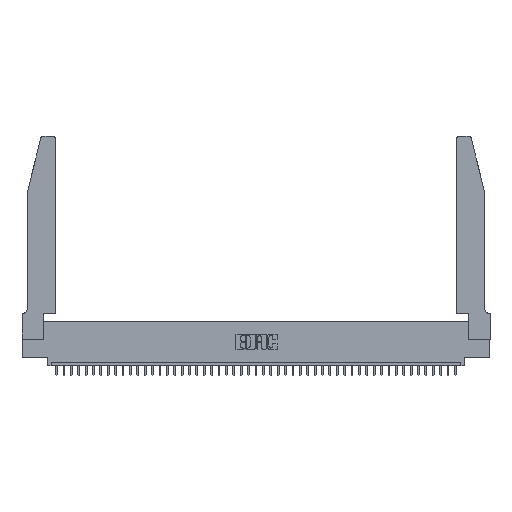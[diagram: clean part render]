
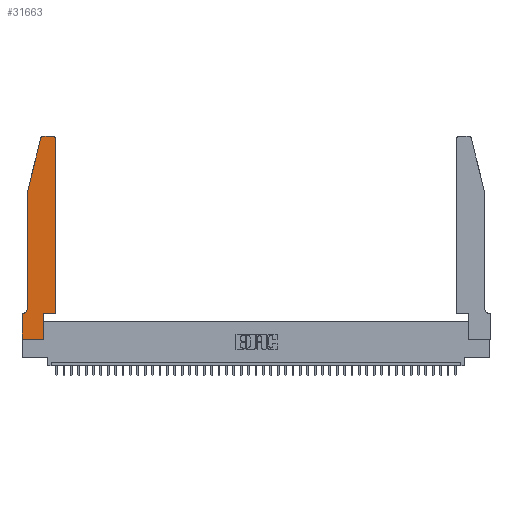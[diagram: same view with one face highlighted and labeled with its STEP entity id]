
A CAD part, top view. The second image highlights one B-rep face of the part: STEP entity #31663.
In plain terms, the highlighted planar face has unit normal (0, 0, 1).
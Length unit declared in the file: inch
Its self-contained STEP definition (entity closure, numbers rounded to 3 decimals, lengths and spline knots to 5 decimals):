
#467 = LINE ( 'NONE', #30379, #32256 ) ;
#498 = EDGE_CURVE ( 'NONE', #43970, #18253, #39390, .T. ) ;
#1003 = FACE_OUTER_BOUND ( 'NONE', #10533, .T. ) ;
#1211 = CIRCLE ( 'NONE', #13735, 0.07 ) ;
#1346 = DIRECTION ( 'NONE',  ( 1., 0., 0. ) ) ;
#2030 = DIRECTION ( 'NONE',  ( 0., 0., -1. ) ) ;
#2126 = EDGE_CURVE ( 'NONE', #4082, #16941, #1211, .T. ) ;
#2591 = CARTESIAN_POINT ( 'NONE',  ( 0.0055, 0.35, 0.37 ) ) ;
#3167 = EDGE_CURVE ( 'NONE', #43345, #43970, #38235, .T. ) ;
#3253 = CARTESIAN_POINT ( 'NONE',  ( 0.2605, 2.75, 0.37 ) ) ;
#3808 = ORIENTED_EDGE ( 'NONE', *, *, #30053, .T. ) ;
#3854 = VECTOR ( 'NONE', #9571, 39.37008 ) ;
#4082 = VERTEX_POINT ( 'NONE', #9560 ) ;
#4664 = DIRECTION ( 'NONE',  ( 0., 1., 0. ) ) ;
#5843 = CARTESIAN_POINT ( 'NONE',  ( 0., 0.35, 0.37 ) ) ;
#6270 = CARTESIAN_POINT ( 'NONE',  ( 0., 0., 0.37 ) ) ;
#9437 = DIRECTION ( 'NONE',  ( 1., 0., 0. ) ) ;
#9560 = CARTESIAN_POINT ( 'NONE',  ( 0.0755, 0.42, 0.37 ) ) ;
#9571 = DIRECTION ( 'NONE',  ( 1., 0., 0. ) ) ;
#10533 = EDGE_LOOP ( 'NONE', ( #23022, #24899, #38651, #12901, #29548, #28961, #37456, #3808, #36586, #33849, #40538, #20449 ) ) ;
#12121 = DIRECTION ( 'NONE',  ( -1., 0., 0. ) ) ;
#12220 = EDGE_CURVE ( 'NONE', #16941, #22167, #467, .T. ) ;
#12901 = ORIENTED_EDGE ( 'NONE', *, *, #14897, .T. ) ;
#13027 = PLANE ( 'NONE',  #43743 ) ;
#13198 = DIRECTION ( 'NONE',  ( 1., 0., 0. ) ) ;
#13690 = CARTESIAN_POINT ( 'NONE',  ( 0.25487, 2.72718, 0.37 ) ) ;
#13735 = AXIS2_PLACEMENT_3D ( 'NONE', #22420, #2030, #12121 ) ;
#13819 = CARTESIAN_POINT ( 'NONE',  ( 0.2865, 0., 0.37 ) ) ;
#14368 = CARTESIAN_POINT ( 'NONE',  ( 0., 0., 0.37 ) ) ;
#14806 = CIRCLE ( 'NONE', #32439, 0.03 ) ;
#14897 = EDGE_CURVE ( 'NONE', #21212, #4082, #32716, .T. ) ;
#15145 = LINE ( 'NONE', #40235, #21542 ) ;
#15285 = CARTESIAN_POINT ( 'NONE',  ( 0., 0., 0.37 ) ) ;
#15328 = CARTESIAN_POINT ( 'NONE',  ( 0.4505, 0.35, 0.37 ) ) ;
#16217 = LINE ( 'NONE', #35385, #42052 ) ;
#16904 = VERTEX_POINT ( 'NONE', #15285 ) ;
#16941 = VERTEX_POINT ( 'NONE', #2591 ) ;
#18173 = LINE ( 'NONE', #21728, #39775 ) ;
#18253 = VERTEX_POINT ( 'NONE', #13690 ) ;
#19038 = LINE ( 'NONE', #20580, #34201 ) ;
#19192 = EDGE_CURVE ( 'NONE', #38780, #36599, #15145, .T. ) ;
#20449 = ORIENTED_EDGE ( 'NONE', *, *, #27461, .T. ) ;
#20580 = CARTESIAN_POINT ( 'NONE',  ( 0.4505, 0.35, 0.37 ) ) ;
#21212 = VERTEX_POINT ( 'NONE', #39791 ) ;
#21542 = VECTOR ( 'NONE', #24767, 39.37008 ) ;
#21728 = CARTESIAN_POINT ( 'NONE',  ( 0.4505, 0.35, 0.37 ) ) ;
#21789 = DIRECTION ( 'NONE',  ( -0.239, -0.971, 0. ) ) ;
#21903 = DIRECTION ( 'NONE',  ( 0., 0., 1. ) ) ;
#22167 = VERTEX_POINT ( 'NONE', #43435 ) ;
#22420 = CARTESIAN_POINT ( 'NONE',  ( 0.0055, 0.42, 0.37 ) ) ;
#22748 = LINE ( 'NONE', #14368, #40016 ) ;
#23022 = ORIENTED_EDGE ( 'NONE', *, *, #3167, .T. ) ;
#23061 = EDGE_CURVE ( 'NONE', #18253, #21212, #16217, .T. ) ;
#23567 = VECTOR ( 'NONE', #38788, 39.37008 ) ;
#24750 = VECTOR ( 'NONE', #27511, 39.37008 ) ;
#24767 = DIRECTION ( 'NONE',  ( 0., 1., 0. ) ) ;
#24899 = ORIENTED_EDGE ( 'NONE', *, *, #498, .T. ) ;
#25700 = CARTESIAN_POINT ( 'NONE',  ( 0.284, 2.72, 0.37 ) ) ;
#26692 = DIRECTION ( 'NONE',  ( 0., 0., 1. ) ) ;
#27052 = DIRECTION ( 'NONE',  ( 1., 0., 0. ) ) ;
#27073 = VERTEX_POINT ( 'NONE', #38041 ) ;
#27461 = EDGE_CURVE ( 'NONE', #27073, #43345, #14806, .T. ) ;
#27511 = DIRECTION ( 'NONE',  ( -1., 0., 0. ) ) ;
#28961 = ORIENTED_EDGE ( 'NONE', *, *, #12220, .T. ) ;
#29004 = CARTESIAN_POINT ( 'NONE',  ( 0.0755, 2., 0.37 ) ) ;
#29036 = VERTEX_POINT ( 'NONE', #15328 ) ;
#29548 = ORIENTED_EDGE ( 'NONE', *, *, #2126, .T. ) ;
#30053 = EDGE_CURVE ( 'NONE', #16904, #38780, #31781, .T. ) ;
#30379 = CARTESIAN_POINT ( 'NONE',  ( 0.0755, 0.35, 0.37 ) ) ;
#31663 = ADVANCED_FACE ( 'NONE', ( #1003 ), #13027, .T. ) ;
#31781 = LINE ( 'NONE', #6270, #3854 ) ;
#32256 = VECTOR ( 'NONE', #33854, 39.37008 ) ;
#32439 = AXIS2_PLACEMENT_3D ( 'NONE', #36181, #26692, #13198 ) ;
#32456 = CARTESIAN_POINT ( 'NONE',  ( 0.2865, 0.35, 0.37 ) ) ;
#32716 = LINE ( 'NONE', #29004, #23567 ) ;
#33849 = ORIENTED_EDGE ( 'NONE', *, *, #35099, .T. ) ;
#33854 = DIRECTION ( 'NONE',  ( -1., 0., 0. ) ) ;
#34201 = VECTOR ( 'NONE', #27052, 39.37008 ) ;
#35099 = EDGE_CURVE ( 'NONE', #36599, #29036, #19038, .T. ) ;
#35385 = CARTESIAN_POINT ( 'NONE',  ( 0.0755, 2., 0.37 ) ) ;
#35882 = EDGE_CURVE ( 'NONE', #22167, #16904, #22748, .T. ) ;
#36181 = CARTESIAN_POINT ( 'NONE',  ( 0.4205, 2.72, 0.37 ) ) ;
#36586 = ORIENTED_EDGE ( 'NONE', *, *, #19192, .T. ) ;
#36599 = VERTEX_POINT ( 'NONE', #32456 ) ;
#37009 = CARTESIAN_POINT ( 'NONE',  ( 0.4205, 2.75, 0.37 ) ) ;
#37456 = ORIENTED_EDGE ( 'NONE', *, *, #35882, .T. ) ;
#38041 = CARTESIAN_POINT ( 'NONE',  ( 0.4505, 2.72, 0.37 ) ) ;
#38235 = LINE ( 'NONE', #3253, #24750 ) ;
#38651 = ORIENTED_EDGE ( 'NONE', *, *, #23061, .T. ) ;
#38696 = AXIS2_PLACEMENT_3D ( 'NONE', #25700, #21903, #1346 ) ;
#38780 = VERTEX_POINT ( 'NONE', #13819 ) ;
#38788 = DIRECTION ( 'NONE',  ( 0., -1., 0. ) ) ;
#39390 = CIRCLE ( 'NONE', #38696, 0.03 ) ;
#39775 = VECTOR ( 'NONE', #4664, 39.37008 ) ;
#39791 = CARTESIAN_POINT ( 'NONE',  ( 0.0755, 2., 0.37 ) ) ;
#40016 = VECTOR ( 'NONE', #41717, 39.37008 ) ;
#40235 = CARTESIAN_POINT ( 'NONE',  ( 0.2865, 0.35, 0.37 ) ) ;
#40538 = ORIENTED_EDGE ( 'NONE', *, *, #43775, .T. ) ;
#41026 = CARTESIAN_POINT ( 'NONE',  ( 0.284, 2.75, 0.37 ) ) ;
#41717 = DIRECTION ( 'NONE',  ( 0., -1., 0. ) ) ;
#42052 = VECTOR ( 'NONE', #21789, 39.37008 ) ;
#43345 = VERTEX_POINT ( 'NONE', #37009 ) ;
#43435 = CARTESIAN_POINT ( 'NONE',  ( 0., 0.35, 0.37 ) ) ;
#43743 = AXIS2_PLACEMENT_3D ( 'NONE', #5843, #43832, #9437 ) ;
#43775 = EDGE_CURVE ( 'NONE', #29036, #27073, #18173, .T. ) ;
#43832 = DIRECTION ( 'NONE',  ( 0., 0., 1. ) ) ;
#43970 = VERTEX_POINT ( 'NONE', #41026 ) ;
